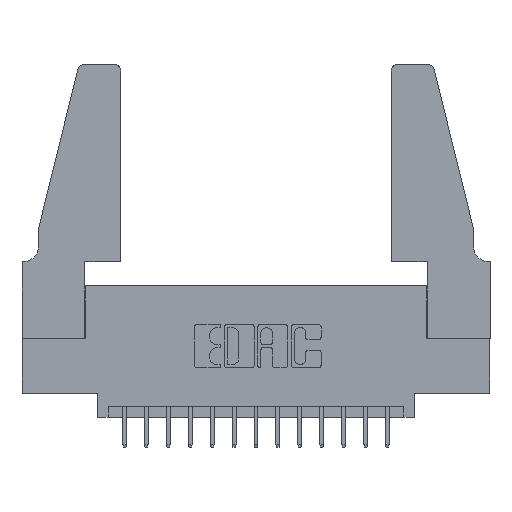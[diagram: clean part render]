
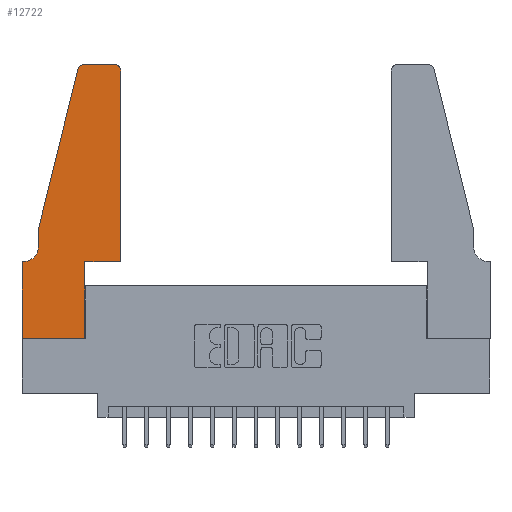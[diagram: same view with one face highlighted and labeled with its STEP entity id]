
A CAD part, top view. The second image highlights one B-rep face of the part: STEP entity #12722.
In plain terms, the highlighted planar face has unit normal (0, 0, 1).
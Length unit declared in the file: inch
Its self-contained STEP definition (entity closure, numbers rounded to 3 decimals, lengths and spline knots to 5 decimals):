
#162 = ORIENTED_EDGE ( 'NONE', *, *, #15375, .T. ) ;
#172 = CIRCLE ( 'NONE', #13499, 0.07 ) ;
#472 = ORIENTED_EDGE ( 'NONE', *, *, #7353, .T. ) ;
#1073 = VECTOR ( 'NONE', #2347, 39.37008 ) ;
#1125 = DIRECTION ( 'NONE',  ( 0., 0., 1. ) ) ;
#1293 = CARTESIAN_POINT ( 'NONE',  ( 0.0055, 0.35, 0.37 ) ) ;
#1327 = CIRCLE ( 'NONE', #11231, 0.03 ) ;
#1336 = ORIENTED_EDGE ( 'NONE', *, *, #3814, .T. ) ;
#1354 = EDGE_CURVE ( 'NONE', #4767, #8413, #1327, .T. ) ;
#1753 = VECTOR ( 'NONE', #6992, 39.37008 ) ;
#1927 = EDGE_CURVE ( 'NONE', #16031, #4767, #15731, .T. ) ;
#2347 = DIRECTION ( 'NONE',  ( 0., -1., 0. ) ) ;
#2798 = EDGE_CURVE ( 'NONE', #5572, #12708, #10752, .T. ) ;
#2835 = LINE ( 'NONE', #14180, #11590 ) ;
#3067 = DIRECTION ( 'NONE',  ( -1., 0., 0. ) ) ;
#3167 = LINE ( 'NONE', #12101, #8676 ) ;
#3401 = CARTESIAN_POINT ( 'NONE',  ( 0., 0., 0.37 ) ) ;
#3500 = EDGE_CURVE ( 'NONE', #3870, #3631, #10471, .T. ) ;
#3631 = VERTEX_POINT ( 'NONE', #4948 ) ;
#3814 = EDGE_CURVE ( 'NONE', #5832, #16031, #12771, .T. ) ;
#3870 = VERTEX_POINT ( 'NONE', #1293 ) ;
#3910 = ORIENTED_EDGE ( 'NONE', *, *, #12241, .T. ) ;
#4044 = ORIENTED_EDGE ( 'NONE', *, *, #10116, .T. ) ;
#4132 = CARTESIAN_POINT ( 'NONE',  ( 0.0755, 0.35, 0.37 ) ) ;
#4518 = CARTESIAN_POINT ( 'NONE',  ( 0.4505, 1.22, 0.37 ) ) ;
#4599 = CARTESIAN_POINT ( 'NONE',  ( 0.4205, 1.22, 0.37 ) ) ;
#4742 = DIRECTION ( 'NONE',  ( 0., 0., 1. ) ) ;
#4767 = VERTEX_POINT ( 'NONE', #8155 ) ;
#4948 = CARTESIAN_POINT ( 'NONE',  ( 0., 0.35, 0.37 ) ) ;
#4952 = CARTESIAN_POINT ( 'NONE',  ( 0.0755, 0.5, 0.37 ) ) ;
#4954 = CARTESIAN_POINT ( 'NONE',  ( 0., 0., 0.37 ) ) ;
#5462 = DIRECTION ( 'NONE',  ( -1., 0., 0. ) ) ;
#5572 = VERTEX_POINT ( 'NONE', #4952 ) ;
#5832 = VERTEX_POINT ( 'NONE', #4518 ) ;
#5875 = CARTESIAN_POINT ( 'NONE',  ( 0.25487, 1.22718, 0.37 ) ) ;
#5885 = VECTOR ( 'NONE', #5962, 39.37008 ) ;
#5962 = DIRECTION ( 'NONE',  ( -0.239, -0.971, 0. ) ) ;
#6153 = VERTEX_POINT ( 'NONE', #8355 ) ;
#6250 = DIRECTION ( 'NONE',  ( 1., 0., 0. ) ) ;
#6906 = LINE ( 'NONE', #13394, #1753 ) ;
#6992 = DIRECTION ( 'NONE',  ( 0., 1., 0. ) ) ;
#7114 = EDGE_CURVE ( 'NONE', #6153, #7881, #2835, .T. ) ;
#7353 = EDGE_CURVE ( 'NONE', #9754, #6153, #3167, .T. ) ;
#7691 = DIRECTION ( 'NONE',  ( 1., 0., 0. ) ) ;
#7776 = DIRECTION ( 'NONE',  ( 1., 0., 0. ) ) ;
#7881 = VERTEX_POINT ( 'NONE', #11459 ) ;
#8155 = CARTESIAN_POINT ( 'NONE',  ( 0.284, 1.25, 0.37 ) ) ;
#8263 = ORIENTED_EDGE ( 'NONE', *, *, #15928, .T. ) ;
#8355 = CARTESIAN_POINT ( 'NONE',  ( 0.2865, 0.35, 0.37 ) ) ;
#8413 = VERTEX_POINT ( 'NONE', #5875 ) ;
#8641 = LINE ( 'NONE', #12308, #5885 ) ;
#8676 = VECTOR ( 'NONE', #15996, 39.37008 ) ;
#9074 = CARTESIAN_POINT ( 'NONE',  ( 0., 0., 0.37 ) ) ;
#9303 = ORIENTED_EDGE ( 'NONE', *, *, #1354, .T. ) ;
#9413 = CARTESIAN_POINT ( 'NONE',  ( 0.2605, 1.25, 0.37 ) ) ;
#9754 = VERTEX_POINT ( 'NONE', #11868 ) ;
#9901 = LINE ( 'NONE', #3401, #1073 ) ;
#10116 = EDGE_CURVE ( 'NONE', #7881, #5832, #6906, .T. ) ;
#10449 = EDGE_LOOP ( 'NONE', ( #10459, #9303, #162, #12448, #13963, #16058, #8263, #3910, #472, #12576, #4044, #1336 ) ) ;
#10459 = ORIENTED_EDGE ( 'NONE', *, *, #1927, .T. ) ;
#10471 = LINE ( 'NONE', #4132, #15958 ) ;
#10560 = CARTESIAN_POINT ( 'NONE',  ( 0.0055, 0.42, 0.37 ) ) ;
#10661 = DIRECTION ( 'NONE',  ( 0., -1., 0. ) ) ;
#10752 = LINE ( 'NONE', #12083, #11010 ) ;
#10984 = VECTOR ( 'NONE', #3067, 39.37008 ) ;
#11010 = VECTOR ( 'NONE', #10661, 39.37008 ) ;
#11231 = AXIS2_PLACEMENT_3D ( 'NONE', #13877, #4742, #15056 ) ;
#11459 = CARTESIAN_POINT ( 'NONE',  ( 0.4505, 0.35, 0.37 ) ) ;
#11590 = VECTOR ( 'NONE', #7776, 39.37008 ) ;
#11646 = DIRECTION ( 'NONE',  ( 0., 0., -1. ) ) ;
#11868 = CARTESIAN_POINT ( 'NONE',  ( 0.2865, 0., 0.37 ) ) ;
#11893 = DIRECTION ( 'NONE',  ( -1., 0., 0. ) ) ;
#12025 = EDGE_CURVE ( 'NONE', #12708, #3870, #172, .T. ) ;
#12083 = CARTESIAN_POINT ( 'NONE',  ( 0.0755, 0.5, 0.37 ) ) ;
#12101 = CARTESIAN_POINT ( 'NONE',  ( 0.2865, 0.35, 0.37 ) ) ;
#12198 = DIRECTION ( 'NONE',  ( 1., 0., 0. ) ) ;
#12228 = AXIS2_PLACEMENT_3D ( 'NONE', #13732, #1125, #6250 ) ;
#12241 = EDGE_CURVE ( 'NONE', #12869, #9754, #16428, .T. ) ;
#12308 = CARTESIAN_POINT ( 'NONE',  ( 0.0755, 0.5, 0.37 ) ) ;
#12368 = DIRECTION ( 'NONE',  ( 0., 0., 1. ) ) ;
#12448 = ORIENTED_EDGE ( 'NONE', *, *, #2798, .T. ) ;
#12576 = ORIENTED_EDGE ( 'NONE', *, *, #7114, .T. ) ;
#12708 = VERTEX_POINT ( 'NONE', #14570 ) ;
#12722 = ADVANCED_FACE ( 'NONE', ( #14653 ), #13416, .T. ) ;
#12771 = CIRCLE ( 'NONE', #16231, 0.03 ) ;
#12790 = CARTESIAN_POINT ( 'NONE',  ( 0.4205, 1.25, 0.37 ) ) ;
#12869 = VERTEX_POINT ( 'NONE', #9074 ) ;
#13394 = CARTESIAN_POINT ( 'NONE',  ( 0.4505, 0.35, 0.37 ) ) ;
#13416 = PLANE ( 'NONE',  #12228 ) ;
#13499 = AXIS2_PLACEMENT_3D ( 'NONE', #10560, #11646, #11893 ) ;
#13732 = CARTESIAN_POINT ( 'NONE',  ( 0., 0.35, 0.37 ) ) ;
#13877 = CARTESIAN_POINT ( 'NONE',  ( 0.284, 1.22, 0.37 ) ) ;
#13963 = ORIENTED_EDGE ( 'NONE', *, *, #12025, .T. ) ;
#14180 = CARTESIAN_POINT ( 'NONE',  ( 0.4505, 0.35, 0.37 ) ) ;
#14305 = VECTOR ( 'NONE', #7691, 39.37008 ) ;
#14570 = CARTESIAN_POINT ( 'NONE',  ( 0.0755, 0.42, 0.37 ) ) ;
#14653 = FACE_OUTER_BOUND ( 'NONE', #10449, .T. ) ;
#15056 = DIRECTION ( 'NONE',  ( 1., 0., 0. ) ) ;
#15375 = EDGE_CURVE ( 'NONE', #8413, #5572, #8641, .T. ) ;
#15731 = LINE ( 'NONE', #9413, #10984 ) ;
#15928 = EDGE_CURVE ( 'NONE', #3631, #12869, #9901, .T. ) ;
#15958 = VECTOR ( 'NONE', #5462, 39.37008 ) ;
#15996 = DIRECTION ( 'NONE',  ( 0., 1., 0. ) ) ;
#16031 = VERTEX_POINT ( 'NONE', #12790 ) ;
#16058 = ORIENTED_EDGE ( 'NONE', *, *, #3500, .T. ) ;
#16231 = AXIS2_PLACEMENT_3D ( 'NONE', #4599, #12368, #12198 ) ;
#16428 = LINE ( 'NONE', #4954, #14305 ) ;
